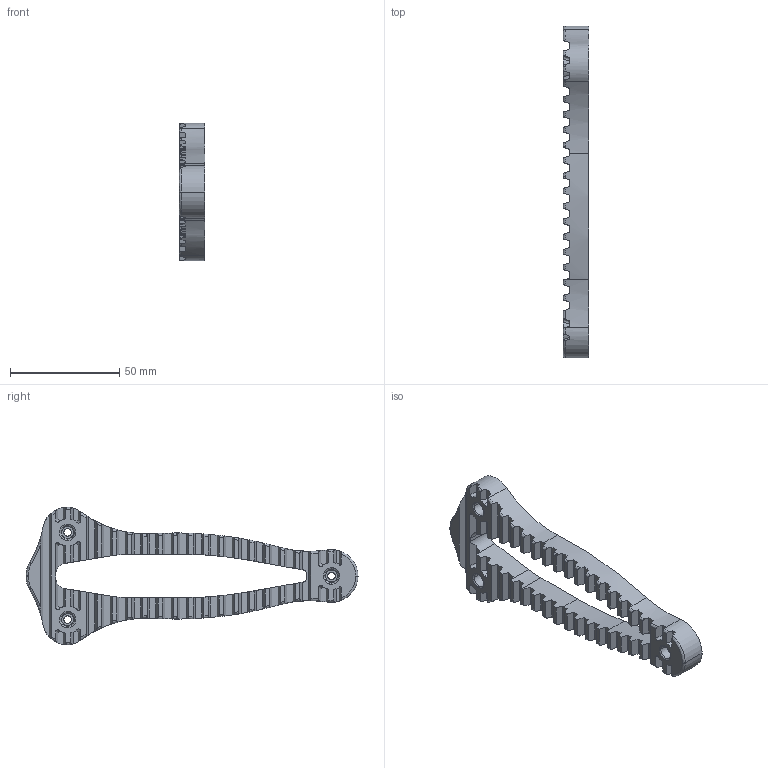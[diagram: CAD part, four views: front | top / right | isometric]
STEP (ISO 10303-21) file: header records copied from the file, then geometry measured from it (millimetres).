
FILE_DESCRIPTION (( 'STEP AP203' ), '1' );
FILE_NAME ('BUTT PLATE.STEP', '2020-09-28T01:12:46', ( '' ), ( '' ), 'SwSTEP 2.0', 'SolidWorks 2019', '' );
FILE_SCHEMA (( 'CONFIG_CONTROL_DESIGN' ));
Length unit declared in the file: millimetre
Products named in the file (1): BUTT PLATE
Bounding box: 11.9 x 152.22 x 63 mm (x, y, z)
Volume: 38566.6 mm3; surface area: 16171.9 mm2
Topology: 1 solids, 1 shells, 294 faces, 864 edges, 574 vertices
Faces by surface type: plane 170, bspline 76, cylinder 48
Entity records: 12357 total; most frequent: CARTESIAN_POINT 5306, ORIENTED_EDGE 1728, DIRECTION 1218, EDGE_CURVE 864, VERTEX_POINT 574, AXIS2_PLACEMENT_3D 450, VECTOR 318, LINE 318
